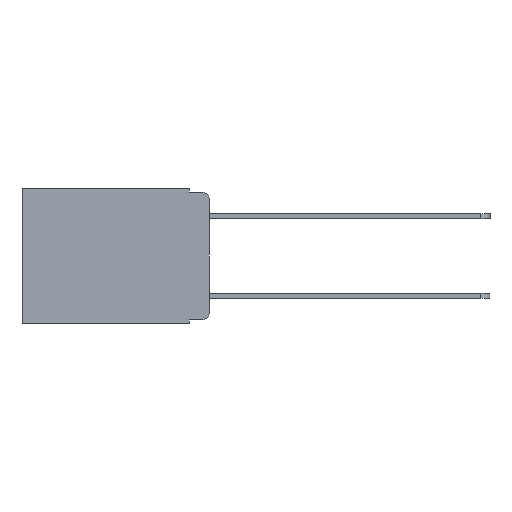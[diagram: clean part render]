
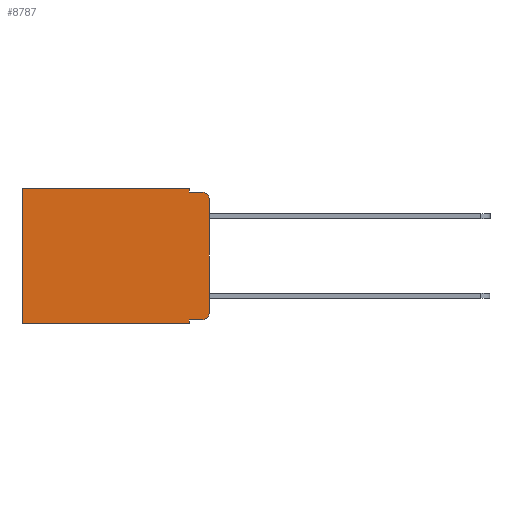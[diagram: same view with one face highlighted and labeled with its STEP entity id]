
A CAD part, left-side view. The second image highlights one B-rep face of the part: STEP entity #8787.
In plain terms, the highlighted planar face has unit normal (-1, 0, 0).
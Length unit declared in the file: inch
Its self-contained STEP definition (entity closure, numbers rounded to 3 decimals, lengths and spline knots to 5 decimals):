
#23 = VERTEX_POINT ( 'NONE', #5731 ) ;
#139 = DIRECTION ( 'NONE',  ( 0., 0., -1. ) ) ;
#189 = CARTESIAN_POINT ( 'NONE',  ( 0.298, 0.473, 0. ) ) ;
#284 = DIRECTION ( 'NONE',  ( -1., 0., 0. ) ) ;
#357 = ORIENTED_EDGE ( 'NONE', *, *, #4428, .T. ) ;
#848 = VERTEX_POINT ( 'NONE', #8655 ) ;
#1068 = LINE ( 'NONE', #7864, #9495 ) ;
#1151 = DIRECTION ( 'NONE',  ( 0., -1., 0. ) ) ;
#1219 = CARTESIAN_POINT ( 'NONE',  ( 0.298, 0.051, -0.333 ) ) ;
#1553 = CARTESIAN_POINT ( 'NONE',  ( 0.298, 0.051, -0.343 ) ) ;
#1581 = FACE_OUTER_BOUND ( 'NONE', #7493, .T. ) ;
#1669 = PLANE ( 'NONE',  #8390 ) ;
#1679 = CARTESIAN_POINT ( 'NONE',  ( 0.298, 0., -0.343 ) ) ;
#1957 = LINE ( 'NONE', #5453, #6180 ) ;
#2021 = ORIENTED_EDGE ( 'NONE', *, *, #4381, .F. ) ;
#2115 = VECTOR ( 'NONE', #5188, 39.37008 ) ;
#2918 = VERTEX_POINT ( 'NONE', #1553 ) ;
#3391 = VERTEX_POINT ( 'NONE', #9917 ) ;
#3530 = DIRECTION ( 'NONE',  ( 0., 0., -1. ) ) ;
#3771 = EDGE_CURVE ( 'NONE', #848, #7200, #10565, .T. ) ;
#3821 = VECTOR ( 'NONE', #1151, 39.37008 ) ;
#3924 = DIRECTION ( 'NONE',  ( 0., 0., -1. ) ) ;
#4067 = LINE ( 'NONE', #7058, #7751 ) ;
#4127 = EDGE_CURVE ( 'NONE', #2918, #6781, #6539, .T. ) ;
#4270 = VERTEX_POINT ( 'NONE', #9225 ) ;
#4337 = EDGE_CURVE ( 'NONE', #10666, #8092, #1957, .T. ) ;
#4365 = EDGE_CURVE ( 'NONE', #10666, #3391, #8215, .T. ) ;
#4381 = EDGE_CURVE ( 'NONE', #23, #3391, #5927, .T. ) ;
#4386 = ORIENTED_EDGE ( 'NONE', *, *, #3771, .T. ) ;
#4397 = EDGE_CURVE ( 'NONE', #848, #23, #4067, .T. ) ;
#4401 = EDGE_CURVE ( 'NONE', #7200, #6781, #6412, .T. ) ;
#4415 = EDGE_CURVE ( 'NONE', #4270, #2918, #1068, .T. ) ;
#4428 = EDGE_CURVE ( 'NONE', #4270, #9110, #7498, .T. ) ;
#4443 = EDGE_CURVE ( 'NONE', #9110, #8092, #5439, .T. ) ;
#4643 = ORIENTED_EDGE ( 'NONE', *, *, #4401, .T. ) ;
#4707 = CARTESIAN_POINT ( 'NONE',  ( 0.298, 0.02, -0.333 ) ) ;
#5188 = DIRECTION ( 'NONE',  ( 0., 1., 0. ) ) ;
#5439 = CIRCLE ( 'NONE', #6680, 0.02 ) ;
#5453 = CARTESIAN_POINT ( 'NONE',  ( 0.298, 0., 0. ) ) ;
#5480 = DIRECTION ( 'NONE',  ( -1., 0., 0. ) ) ;
#5511 = DIRECTION ( 'NONE',  ( 0., 0., -1. ) ) ;
#5568 = CARTESIAN_POINT ( 'NONE',  ( 0.298, 0.02, -0.313 ) ) ;
#5664 = VECTOR ( 'NONE', #7122, 39.37008 ) ;
#5718 = ORIENTED_EDGE ( 'NONE', *, *, #4337, .F. ) ;
#5731 = CARTESIAN_POINT ( 'NONE',  ( 0.298, 0.051, -0.01 ) ) ;
#5927 = LINE ( 'NONE', #8552, #3821 ) ;
#5935 = CARTESIAN_POINT ( 'NONE',  ( 0.298, 0.473, -0.343 ) ) ;
#5984 = ORIENTED_EDGE ( 'NONE', *, *, #4365, .T. ) ;
#6051 = AXIS2_PLACEMENT_3D ( 'NONE', #10063, #5480, #139 ) ;
#6180 = VECTOR ( 'NONE', #6247, 39.37008 ) ;
#6247 = DIRECTION ( 'NONE',  ( 0., 0., -1. ) ) ;
#6305 = VECTOR ( 'NONE', #7564, 39.37008 ) ;
#6379 = DIRECTION ( 'NONE',  ( 0., 0., -1. ) ) ;
#6412 = LINE ( 'NONE', #189, #7984 ) ;
#6539 = LINE ( 'NONE', #1679, #2115 ) ;
#6680 = AXIS2_PLACEMENT_3D ( 'NONE', #5568, #284, #6379 ) ;
#6702 = ORIENTED_EDGE ( 'NONE', *, *, #4415, .F. ) ;
#6781 = VERTEX_POINT ( 'NONE', #5935 ) ;
#6789 = CARTESIAN_POINT ( 'NONE',  ( 0.298, 0., 0. ) ) ;
#7058 = CARTESIAN_POINT ( 'NONE',  ( 0.298, 0.051, 0. ) ) ;
#7122 = DIRECTION ( 'NONE',  ( 0., -1., 0. ) ) ;
#7200 = VERTEX_POINT ( 'NONE', #7217 ) ;
#7217 = CARTESIAN_POINT ( 'NONE',  ( 0.298, 0.473, 0. ) ) ;
#7326 = CARTESIAN_POINT ( 'NONE',  ( 0.298, 0., -0.03 ) ) ;
#7486 = CARTESIAN_POINT ( 'NONE',  ( 0.298, 0., 0. ) ) ;
#7493 = EDGE_LOOP ( 'NONE', ( #5718, #5984, #2021, #8263, #4386, #4643, #8507, #6702, #357, #9221 ) ) ;
#7498 = LINE ( 'NONE', #1219, #5664 ) ;
#7564 = DIRECTION ( 'NONE',  ( 0., 1., 0. ) ) ;
#7751 = VECTOR ( 'NONE', #5511, 39.37008 ) ;
#7864 = CARTESIAN_POINT ( 'NONE',  ( 0.298, 0.051, 0. ) ) ;
#7984 = VECTOR ( 'NONE', #3924, 39.37008 ) ;
#8092 = VERTEX_POINT ( 'NONE', #9636 ) ;
#8215 = CIRCLE ( 'NONE', #6051, 0.02 ) ;
#8250 = DIRECTION ( 'NONE',  ( 1., 0., 0. ) ) ;
#8263 = ORIENTED_EDGE ( 'NONE', *, *, #4397, .F. ) ;
#8390 = AXIS2_PLACEMENT_3D ( 'NONE', #7486, #8250, #3530 ) ;
#8507 = ORIENTED_EDGE ( 'NONE', *, *, #4127, .F. ) ;
#8552 = CARTESIAN_POINT ( 'NONE',  ( 0.298, 0.051, -0.01 ) ) ;
#8612 = DIRECTION ( 'NONE',  ( 0., 0., -1. ) ) ;
#8655 = CARTESIAN_POINT ( 'NONE',  ( 0.298, 0.051, 0. ) ) ;
#8787 = ADVANCED_FACE ( 'NONE', ( #1581 ), #1669, .F. ) ;
#9110 = VERTEX_POINT ( 'NONE', #4707 ) ;
#9221 = ORIENTED_EDGE ( 'NONE', *, *, #4443, .T. ) ;
#9225 = CARTESIAN_POINT ( 'NONE',  ( 0.298, 0.051, -0.333 ) ) ;
#9495 = VECTOR ( 'NONE', #8612, 39.37008 ) ;
#9636 = CARTESIAN_POINT ( 'NONE',  ( 0.298, 0., -0.313 ) ) ;
#9917 = CARTESIAN_POINT ( 'NONE',  ( 0.298, 0.02, -0.01 ) ) ;
#10063 = CARTESIAN_POINT ( 'NONE',  ( 0.298, 0.02, -0.03 ) ) ;
#10565 = LINE ( 'NONE', #6789, #6305 ) ;
#10666 = VERTEX_POINT ( 'NONE', #7326 ) ;
